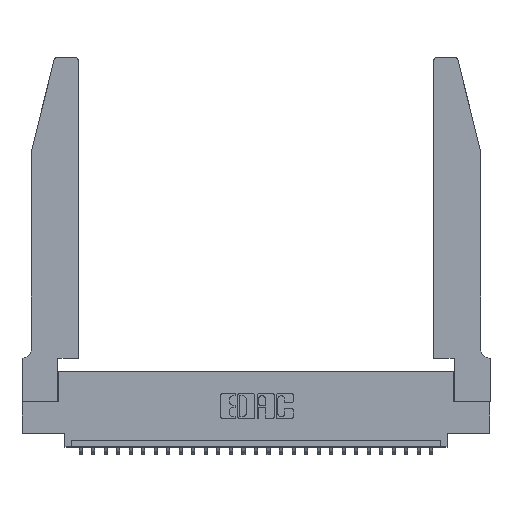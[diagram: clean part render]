
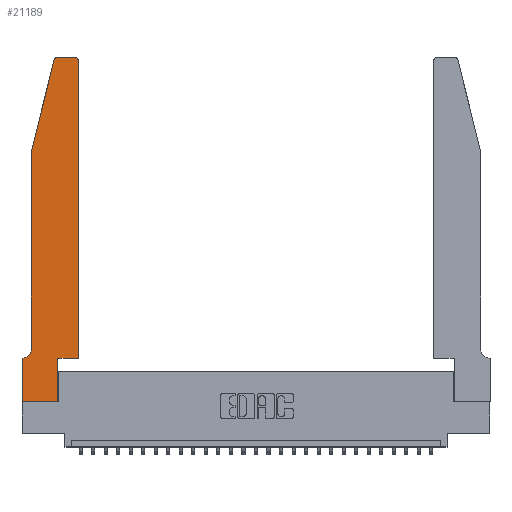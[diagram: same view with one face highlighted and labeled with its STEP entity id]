
A CAD part, top view. The second image highlights one B-rep face of the part: STEP entity #21189.
In plain terms, the highlighted planar face has unit normal (0, 0, 1).
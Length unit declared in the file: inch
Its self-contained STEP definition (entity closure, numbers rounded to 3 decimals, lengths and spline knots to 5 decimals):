
#418 = ORIENTED_EDGE ( 'NONE', *, *, #21138, .T. ) ;
#437 = VERTEX_POINT ( 'NONE', #26405 ) ;
#611 = VERTEX_POINT ( 'NONE', #11211 ) ;
#1406 = VECTOR ( 'NONE', #11087, 39.37008 ) ;
#1927 = ORIENTED_EDGE ( 'NONE', *, *, #18319, .T. ) ;
#2388 = LINE ( 'NONE', #18783, #20310 ) ;
#2505 = VERTEX_POINT ( 'NONE', #19127 ) ;
#2585 = VECTOR ( 'NONE', #14295, 39.37008 ) ;
#2588 = ORIENTED_EDGE ( 'NONE', *, *, #15929, .T. ) ;
#2957 = DIRECTION ( 'NONE',  ( 0., 0., 1. ) ) ;
#2980 = DIRECTION ( 'NONE',  ( 1., 0., 0. ) ) ;
#3213 = CARTESIAN_POINT ( 'NONE',  ( 0., 0., 0.37 ) ) ;
#3294 = CARTESIAN_POINT ( 'NONE',  ( 0.0755, 2., 0.37 ) ) ;
#4142 = LINE ( 'NONE', #15231, #11725 ) ;
#4283 = DIRECTION ( 'NONE',  ( 1., 0., 0. ) ) ;
#4418 = AXIS2_PLACEMENT_3D ( 'NONE', #14243, #2957, #4283 ) ;
#4816 = CIRCLE ( 'NONE', #19597, 0.07 ) ;
#4887 = CARTESIAN_POINT ( 'NONE',  ( 0.4205, 2.75, 0.37 ) ) ;
#5225 = VERTEX_POINT ( 'NONE', #3213 ) ;
#6615 = VERTEX_POINT ( 'NONE', #25312 ) ;
#6810 = DIRECTION ( 'NONE',  ( 0., 1., 0. ) ) ;
#7201 = LINE ( 'NONE', #25839, #1406 ) ;
#7434 = ORIENTED_EDGE ( 'NONE', *, *, #17584, .T. ) ;
#7438 = CARTESIAN_POINT ( 'NONE',  ( 0.284, 2.72, 0.37 ) ) ;
#7711 = EDGE_CURVE ( 'NONE', #24569, #24933, #2388, .T. ) ;
#7996 = DIRECTION ( 'NONE',  ( 0., 0., -1. ) ) ;
#8762 = CARTESIAN_POINT ( 'NONE',  ( 0.2865, 0.35, 0.37 ) ) ;
#9125 = DIRECTION ( 'NONE',  ( 0., 0., 1. ) ) ;
#9725 = VERTEX_POINT ( 'NONE', #4887 ) ;
#9872 = DIRECTION ( 'NONE',  ( -1., 0., 0. ) ) ;
#10034 = LINE ( 'NONE', #3294, #25550 ) ;
#10098 = PLANE ( 'NONE',  #28405 ) ;
#10252 = DIRECTION ( 'NONE',  ( -1., 0., 0. ) ) ;
#10345 = CARTESIAN_POINT ( 'NONE',  ( 0.0755, 0.42, 0.37 ) ) ;
#10385 = DIRECTION ( 'NONE',  ( 0., 0., 1. ) ) ;
#11087 = DIRECTION ( 'NONE',  ( -1., 0., 0. ) ) ;
#11211 = CARTESIAN_POINT ( 'NONE',  ( 0.0755, 2., 0.37 ) ) ;
#11725 = VECTOR ( 'NONE', #15406, 39.37008 ) ;
#11737 = CIRCLE ( 'NONE', #4418, 0.03 ) ;
#11965 = EDGE_CURVE ( 'NONE', #9725, #17611, #7201, .T. ) ;
#12374 = CARTESIAN_POINT ( 'NONE',  ( 0.0055, 0.42, 0.37 ) ) ;
#12470 = ORIENTED_EDGE ( 'NONE', *, *, #11965, .T. ) ;
#12558 = LINE ( 'NONE', #26635, #20847 ) ;
#12671 = CARTESIAN_POINT ( 'NONE',  ( 0.25487, 2.72718, 0.37 ) ) ;
#14243 = CARTESIAN_POINT ( 'NONE',  ( 0.4205, 2.72, 0.37 ) ) ;
#14295 = DIRECTION ( 'NONE',  ( 0., -1., 0. ) ) ;
#14354 = DIRECTION ( 'NONE',  ( 1., 0., 0. ) ) ;
#14394 = CARTESIAN_POINT ( 'NONE',  ( 0.284, 2.75, 0.37 ) ) ;
#14396 = CARTESIAN_POINT ( 'NONE',  ( 0., 0., 0.37 ) ) ;
#15122 = AXIS2_PLACEMENT_3D ( 'NONE', #7438, #9125, #2980 ) ;
#15126 = ORIENTED_EDGE ( 'NONE', *, *, #15472, .T. ) ;
#15231 = CARTESIAN_POINT ( 'NONE',  ( 0.0755, 2., 0.37 ) ) ;
#15267 = LINE ( 'NONE', #25451, #20441 ) ;
#15406 = DIRECTION ( 'NONE',  ( -0.239, -0.971, 0. ) ) ;
#15472 = EDGE_CURVE ( 'NONE', #16782, #26514, #4816, .T. ) ;
#15711 = LINE ( 'NONE', #14396, #2585 ) ;
#15859 = CARTESIAN_POINT ( 'NONE',  ( 0.4505, 0.35, 0.37 ) ) ;
#15929 = EDGE_CURVE ( 'NONE', #2505, #9725, #11737, .T. ) ;
#16106 = EDGE_CURVE ( 'NONE', #6615, #24569, #27922, .T. ) ;
#16142 = FACE_OUTER_BOUND ( 'NONE', #20965, .T. ) ;
#16539 = CARTESIAN_POINT ( 'NONE',  ( 0.0755, 0.35, 0.37 ) ) ;
#16758 = ORIENTED_EDGE ( 'NONE', *, *, #16106, .T. ) ;
#16782 = VERTEX_POINT ( 'NONE', #10345 ) ;
#17584 = EDGE_CURVE ( 'NONE', #611, #16782, #10034, .T. ) ;
#17611 = VERTEX_POINT ( 'NONE', #14394 ) ;
#18319 = EDGE_CURVE ( 'NONE', #5225, #6615, #15267, .T. ) ;
#18783 = CARTESIAN_POINT ( 'NONE',  ( 0.4505, 0.35, 0.37 ) ) ;
#18953 = ORIENTED_EDGE ( 'NONE', *, *, #26114, .T. ) ;
#18975 = DIRECTION ( 'NONE',  ( 1., 0., 0. ) ) ;
#19048 = LINE ( 'NONE', #16539, #25944 ) ;
#19127 = CARTESIAN_POINT ( 'NONE',  ( 0.4505, 2.72, 0.37 ) ) ;
#19597 = AXIS2_PLACEMENT_3D ( 'NONE', #12374, #7996, #10252 ) ;
#19611 = CIRCLE ( 'NONE', #15122, 0.03 ) ;
#19731 = CARTESIAN_POINT ( 'NONE',  ( 0.2865, 0.35, 0.37 ) ) ;
#19962 = CARTESIAN_POINT ( 'NONE',  ( 0.0055, 0.35, 0.37 ) ) ;
#20206 = EDGE_CURVE ( 'NONE', #21966, #611, #4142, .T. ) ;
#20310 = VECTOR ( 'NONE', #21504, 39.37008 ) ;
#20441 = VECTOR ( 'NONE', #18975, 39.37008 ) ;
#20847 = VECTOR ( 'NONE', #6810, 39.37008 ) ;
#20965 = EDGE_LOOP ( 'NONE', ( #12470, #418, #27117, #7434, #15126, #27519, #23561, #1927, #16758, #22748, #18953, #2588 ) ) ;
#21138 = EDGE_CURVE ( 'NONE', #17611, #21966, #19611, .T. ) ;
#21189 = ADVANCED_FACE ( 'NONE', ( #16142 ), #10098, .T. ) ;
#21504 = DIRECTION ( 'NONE',  ( 1., 0., 0. ) ) ;
#21966 = VERTEX_POINT ( 'NONE', #12671 ) ;
#22748 = ORIENTED_EDGE ( 'NONE', *, *, #7711, .T. ) ;
#23561 = ORIENTED_EDGE ( 'NONE', *, *, #25499, .T. ) ;
#24569 = VERTEX_POINT ( 'NONE', #19731 ) ;
#24849 = VECTOR ( 'NONE', #28540, 39.37008 ) ;
#24933 = VERTEX_POINT ( 'NONE', #15859 ) ;
#25312 = CARTESIAN_POINT ( 'NONE',  ( 0.2865, 0., 0.37 ) ) ;
#25451 = CARTESIAN_POINT ( 'NONE',  ( 0., 0., 0.37 ) ) ;
#25499 = EDGE_CURVE ( 'NONE', #437, #5225, #15711, .T. ) ;
#25550 = VECTOR ( 'NONE', #25593, 39.37008 ) ;
#25593 = DIRECTION ( 'NONE',  ( 0., -1., 0. ) ) ;
#25839 = CARTESIAN_POINT ( 'NONE',  ( 0.2605, 2.75, 0.37 ) ) ;
#25944 = VECTOR ( 'NONE', #9872, 39.37008 ) ;
#26114 = EDGE_CURVE ( 'NONE', #24933, #2505, #12558, .T. ) ;
#26405 = CARTESIAN_POINT ( 'NONE',  ( 0., 0.35, 0.37 ) ) ;
#26514 = VERTEX_POINT ( 'NONE', #19962 ) ;
#26635 = CARTESIAN_POINT ( 'NONE',  ( 0.4505, 0.35, 0.37 ) ) ;
#27117 = ORIENTED_EDGE ( 'NONE', *, *, #20206, .T. ) ;
#27418 = EDGE_CURVE ( 'NONE', #26514, #437, #19048, .T. ) ;
#27519 = ORIENTED_EDGE ( 'NONE', *, *, #27418, .T. ) ;
#27752 = CARTESIAN_POINT ( 'NONE',  ( 0., 0.35, 0.37 ) ) ;
#27922 = LINE ( 'NONE', #8762, #24849 ) ;
#28405 = AXIS2_PLACEMENT_3D ( 'NONE', #27752, #10385, #14354 ) ;
#28540 = DIRECTION ( 'NONE',  ( 0., 1., 0. ) ) ;
